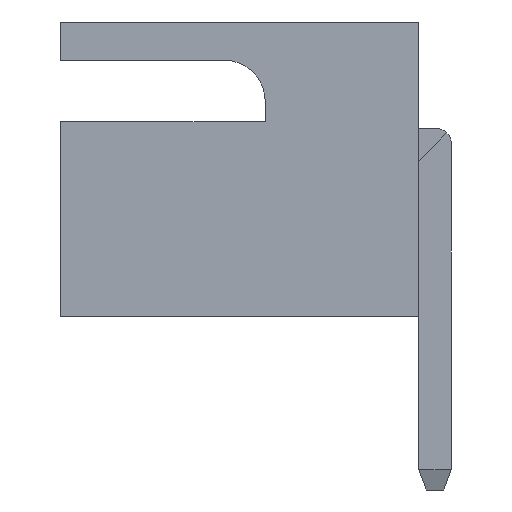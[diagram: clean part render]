
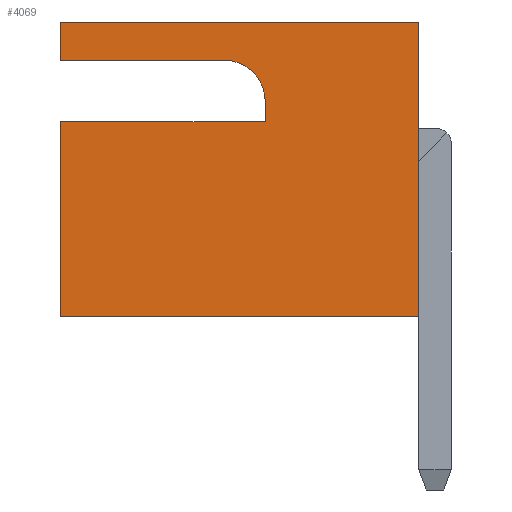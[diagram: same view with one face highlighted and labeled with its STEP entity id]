
A CAD part, left-side view. The second image highlights one B-rep face of the part: STEP entity #4069.
In plain terms, the highlighted planar face has unit normal (-1, 0, 0).
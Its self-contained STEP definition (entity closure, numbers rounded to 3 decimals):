
#139 = CARTESIAN_POINT ( 'NONE',  ( -10., 3.8, 2.125 ) ) ;
#144 = CARTESIAN_POINT ( 'NONE',  ( -10., 7., 2.125 ) ) ;
#381 = CARTESIAN_POINT ( 'NONE',  ( -10., 0., -2.875 ) ) ;
#428 = VECTOR ( 'NONE', #1338, 1000. ) ;
#461 = CARTESIAN_POINT ( 'NONE',  ( -10., 7., -2.875 ) ) ;
#470 = ORIENTED_EDGE ( 'NONE', *, *, #1800, .F. ) ;
#479 = CARTESIAN_POINT ( 'NONE',  ( -10., 7., -2.875 ) ) ;
#490 = DIRECTION ( 'NONE',  ( 0., -1., 0. ) ) ;
#504 = DIRECTION ( 'NONE',  ( 1., 0., 0. ) ) ;
#518 = EDGE_CURVE ( 'NONE', #3884, #3122, #3890, .T. ) ;
#533 = CIRCLE ( 'NONE', #1628, 0.8 ) ;
#819 = CARTESIAN_POINT ( 'NONE',  ( -10., 3., 0.925 ) ) ;
#938 = VECTOR ( 'NONE', #3058, 1000. ) ;
#1003 = CARTESIAN_POINT ( 'NONE',  ( -10., 0., -2.875 ) ) ;
#1067 = EDGE_CURVE ( 'NONE', #2443, #1962, #3781, .T. ) ;
#1145 = PLANE ( 'NONE',  #3283 ) ;
#1160 = CARTESIAN_POINT ( 'NONE',  ( -10., 7., -2.875 ) ) ;
#1171 = ORIENTED_EDGE ( 'NONE', *, *, #1684, .F. ) ;
#1211 = DIRECTION ( 'NONE',  ( 0., 1., 0. ) ) ;
#1215 = FACE_OUTER_BOUND ( 'NONE', #1597, .T. ) ;
#1338 = DIRECTION ( 'NONE',  ( 0., -1., 0. ) ) ;
#1597 = EDGE_LOOP ( 'NONE', ( #2372, #1604, #1788, #3405, #3695, #1171, #2820, #3172, #470 ) ) ;
#1604 = ORIENTED_EDGE ( 'NONE', *, *, #1067, .T. ) ;
#1621 = CARTESIAN_POINT ( 'NONE',  ( -10., 3.8, 1.325 ) ) ;
#1628 = AXIS2_PLACEMENT_3D ( 'NONE', #1621, #4150, #3026 ) ;
#1682 = CARTESIAN_POINT ( 'NONE',  ( -10., 3., 1.325 ) ) ;
#1684 = EDGE_CURVE ( 'NONE', #3884, #4433, #2983, .T. ) ;
#1788 = ORIENTED_EDGE ( 'NONE', *, *, #3488, .T. ) ;
#1800 = EDGE_CURVE ( 'NONE', #3269, #3782, #4316, .T. ) ;
#1866 = VECTOR ( 'NONE', #2162, 1000. ) ;
#1872 = DIRECTION ( 'NONE',  ( 0., 0., 1. ) ) ;
#1962 = VERTEX_POINT ( 'NONE', #139 ) ;
#1968 = EDGE_CURVE ( 'NONE', #2269, #3035, #4184, .T. ) ;
#1980 = DIRECTION ( 'NONE',  ( 0., 0., -1. ) ) ;
#2041 = VECTOR ( 'NONE', #3418, 1000. ) ;
#2162 = DIRECTION ( 'NONE',  ( 0., -1., 0. ) ) ;
#2269 = VERTEX_POINT ( 'NONE', #2534 ) ;
#2372 = ORIENTED_EDGE ( 'NONE', *, *, #3040, .F. ) ;
#2443 = VERTEX_POINT ( 'NONE', #4436 ) ;
#2492 = CARTESIAN_POINT ( 'NONE',  ( -10., 7., -2.875 ) ) ;
#2534 = CARTESIAN_POINT ( 'NONE',  ( -10., 3., 1.325 ) ) ;
#2613 = CARTESIAN_POINT ( 'NONE',  ( -10., 0., 2.875 ) ) ;
#2619 = DIRECTION ( 'NONE',  ( 0., 0., 1. ) ) ;
#2624 = VECTOR ( 'NONE', #2619, 1000. ) ;
#2706 = LINE ( 'NONE', #461, #2041 ) ;
#2820 = ORIENTED_EDGE ( 'NONE', *, *, #518, .T. ) ;
#2944 = VECTOR ( 'NONE', #490, 1000. ) ;
#2983 = LINE ( 'NONE', #1160, #2624 ) ;
#3008 = CARTESIAN_POINT ( 'NONE',  ( -10., 7., 2.875 ) ) ;
#3026 = DIRECTION ( 'NONE',  ( 0., 0., -1. ) ) ;
#3035 = VERTEX_POINT ( 'NONE', #819 ) ;
#3040 = EDGE_CURVE ( 'NONE', #2443, #3269, #2706, .T. ) ;
#3058 = DIRECTION ( 'NONE',  ( 0., 0., -1. ) ) ;
#3122 = VERTEX_POINT ( 'NONE', #1003 ) ;
#3172 = ORIENTED_EDGE ( 'NONE', *, *, #4040, .T. ) ;
#3269 = VERTEX_POINT ( 'NONE', #3008 ) ;
#3283 = AXIS2_PLACEMENT_3D ( 'NONE', #479, #504, #1980 ) ;
#3387 = CARTESIAN_POINT ( 'NONE',  ( -10., 7., 0.925 ) ) ;
#3405 = ORIENTED_EDGE ( 'NONE', *, *, #1968, .T. ) ;
#3418 = DIRECTION ( 'NONE',  ( 0., 0., 1. ) ) ;
#3453 = EDGE_CURVE ( 'NONE', #3035, #4433, #3745, .T. ) ;
#3488 = EDGE_CURVE ( 'NONE', #1962, #2269, #533, .T. ) ;
#3595 = CARTESIAN_POINT ( 'NONE',  ( -10., 7., 2.875 ) ) ;
#3677 = LINE ( 'NONE', #381, #4348 ) ;
#3695 = ORIENTED_EDGE ( 'NONE', *, *, #3453, .T. ) ;
#3745 = LINE ( 'NONE', #3387, #4001 ) ;
#3781 = LINE ( 'NONE', #144, #2944 ) ;
#3782 = VERTEX_POINT ( 'NONE', #2613 ) ;
#3884 = VERTEX_POINT ( 'NONE', #2492 ) ;
#3890 = LINE ( 'NONE', #4268, #428 ) ;
#4001 = VECTOR ( 'NONE', #1211, 1000. ) ;
#4040 = EDGE_CURVE ( 'NONE', #3122, #3782, #3677, .T. ) ;
#4069 = ADVANCED_FACE ( 'NONE', ( #1215 ), #1145, .F. ) ;
#4150 = DIRECTION ( 'NONE',  ( 1., 0., 0. ) ) ;
#4184 = LINE ( 'NONE', #1682, #938 ) ;
#4268 = CARTESIAN_POINT ( 'NONE',  ( -10., 7., -2.875 ) ) ;
#4316 = LINE ( 'NONE', #3595, #1866 ) ;
#4348 = VECTOR ( 'NONE', #1872, 1000. ) ;
#4433 = VERTEX_POINT ( 'NONE', #4666 ) ;
#4436 = CARTESIAN_POINT ( 'NONE',  ( -10., 7., 2.125 ) ) ;
#4666 = CARTESIAN_POINT ( 'NONE',  ( -10., 7., 0.925 ) ) ;
